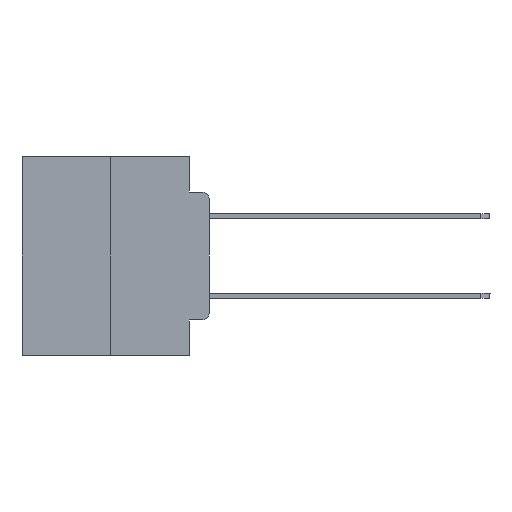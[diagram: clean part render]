
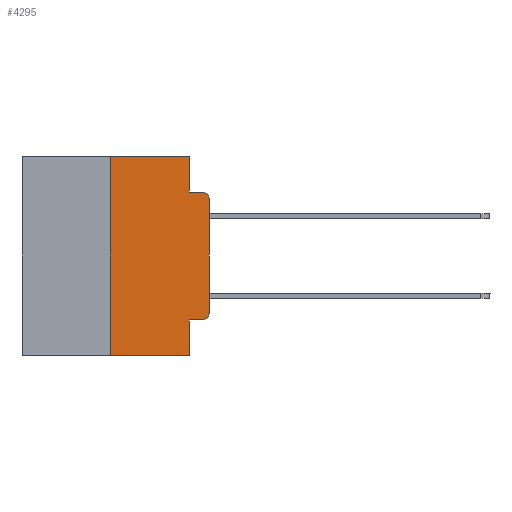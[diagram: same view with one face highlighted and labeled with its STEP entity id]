
A CAD part, left-side view. The second image highlights one B-rep face of the part: STEP entity #4295.
In plain terms, the highlighted planar face has unit normal (-1, 0, 0).
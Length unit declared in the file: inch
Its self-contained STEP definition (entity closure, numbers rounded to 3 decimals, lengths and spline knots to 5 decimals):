
#79 = AXIS2_PLACEMENT_3D ( 'NONE', #15907, #11477, #24116 ) ;
#836 = EDGE_CURVE ( 'NONE', #24686, #2357, #16150, .T. ) ;
#2034 = DIRECTION ( 'NONE',  ( 0., -1., 0. ) ) ;
#2182 = CARTESIAN_POINT ( 'NONE',  ( 0., 0.25, 0. ) ) ;
#2357 = VERTEX_POINT ( 'NONE', #9344 ) ;
#2417 = VECTOR ( 'NONE', #21126, 39.37008 ) ;
#2919 = VECTOR ( 'NONE', #4242, 39.37008 ) ;
#3488 = CIRCLE ( 'NONE', #19843, 0.02 ) ;
#3602 = ORIENTED_EDGE ( 'NONE', *, *, #19411, .F. ) ;
#3713 = DIRECTION ( 'NONE',  ( 0., 0., 1. ) ) ;
#3742 = DIRECTION ( 'NONE',  ( 0., -1., 0. ) ) ;
#3765 = DIRECTION ( 'NONE',  ( 1., 0., 0. ) ) ;
#4242 = DIRECTION ( 'NONE',  ( 0., 0., -1. ) ) ;
#4295 = ADVANCED_FACE ( 'NONE', ( #25111 ), #20653, .F. ) ;
#4565 = VERTEX_POINT ( 'NONE', #24387 ) ;
#4983 = CARTESIAN_POINT ( 'NONE',  ( 0., 0.473, -0.5 ) ) ;
#5387 = CARTESIAN_POINT ( 'NONE',  ( 0., 0., 0. ) ) ;
#5535 = VERTEX_POINT ( 'NONE', #21459 ) ;
#5668 = ORIENTED_EDGE ( 'NONE', *, *, #836, .T. ) ;
#6064 = ORIENTED_EDGE ( 'NONE', *, *, #25754, .T. ) ;
#6255 = ORIENTED_EDGE ( 'NONE', *, *, #13074, .F. ) ;
#6963 = EDGE_CURVE ( 'NONE', #5535, #24871, #11880, .T. ) ;
#7168 = EDGE_CURVE ( 'NONE', #12457, #4565, #27125, .T. ) ;
#7212 = VERTEX_POINT ( 'NONE', #16848 ) ;
#7243 = VECTOR ( 'NONE', #3713, 39.37008 ) ;
#7397 = CARTESIAN_POINT ( 'NONE',  ( 0., 0., -0.1085 ) ) ;
#8178 = VECTOR ( 'NONE', #10061, 39.37008 ) ;
#8630 = LINE ( 'NONE', #19157, #16765 ) ;
#8687 = ORIENTED_EDGE ( 'NONE', *, *, #22724, .T. ) ;
#9344 = CARTESIAN_POINT ( 'NONE',  ( 0., 0.051, -0.5 ) ) ;
#9459 = CARTESIAN_POINT ( 'NONE',  ( 0., 0.051, -0.4115 ) ) ;
#9720 = EDGE_CURVE ( 'NONE', #24686, #15168, #8630, .T. ) ;
#9820 = EDGE_CURVE ( 'NONE', #12457, #2357, #15139, .T. ) ;
#10061 = DIRECTION ( 'NONE',  ( 0., -1., 0. ) ) ;
#10525 = EDGE_CURVE ( 'NONE', #14045, #7212, #22675, .T. ) ;
#11477 = DIRECTION ( 'NONE',  ( -1., 0., 0. ) ) ;
#11880 = LINE ( 'NONE', #5387, #7243 ) ;
#12050 = LINE ( 'NONE', #18420, #20380 ) ;
#12457 = VERTEX_POINT ( 'NONE', #9459 ) ;
#12763 = ORIENTED_EDGE ( 'NONE', *, *, #7168, .T. ) ;
#13074 = EDGE_CURVE ( 'NONE', #15168, #25402, #12050, .T. ) ;
#14045 = VERTEX_POINT ( 'NONE', #24645 ) ;
#14866 = CARTESIAN_POINT ( 'NONE',  ( 0., 0.051, 0. ) ) ;
#15139 = LINE ( 'NONE', #14866, #22537 ) ;
#15168 = VERTEX_POINT ( 'NONE', #2182 ) ;
#15572 = ORIENTED_EDGE ( 'NONE', *, *, #9820, .F. ) ;
#15907 = CARTESIAN_POINT ( 'NONE',  ( 0., 0.02, -0.3915 ) ) ;
#15971 = ORIENTED_EDGE ( 'NONE', *, *, #6963, .T. ) ;
#16150 = LINE ( 'NONE', #4983, #8178 ) ;
#16385 = AXIS2_PLACEMENT_3D ( 'NONE', #25237, #3765, #27173 ) ;
#16717 = CARTESIAN_POINT ( 'NONE',  ( 0., 0.051, -0.4115 ) ) ;
#16765 = VECTOR ( 'NONE', #23182, 39.37008 ) ;
#16848 = CARTESIAN_POINT ( 'NONE',  ( 0., 0.02, -0.0885 ) ) ;
#17257 = LINE ( 'NONE', #23227, #2919 ) ;
#18420 = CARTESIAN_POINT ( 'NONE',  ( 0., 0.473, 0. ) ) ;
#19157 = CARTESIAN_POINT ( 'NONE',  ( 0., 0.25, 0. ) ) ;
#19411 = EDGE_CURVE ( 'NONE', #25402, #14045, #17257, .T. ) ;
#19843 = AXIS2_PLACEMENT_3D ( 'NONE', #20330, #26729, #26458 ) ;
#20330 = CARTESIAN_POINT ( 'NONE',  ( 0., 0.02, -0.1085 ) ) ;
#20380 = VECTOR ( 'NONE', #3742, 39.37008 ) ;
#20512 = VECTOR ( 'NONE', #2034, 39.37008 ) ;
#20653 = PLANE ( 'NONE',  #16385 ) ;
#20917 = CARTESIAN_POINT ( 'NONE',  ( 0., 0.051, 0. ) ) ;
#21126 = DIRECTION ( 'NONE',  ( 0., -1., 0. ) ) ;
#21459 = CARTESIAN_POINT ( 'NONE',  ( 0., 0., -0.3915 ) ) ;
#21768 = CIRCLE ( 'NONE', #79, 0.02 ) ;
#22537 = VECTOR ( 'NONE', #23318, 39.37008 ) ;
#22675 = LINE ( 'NONE', #27106, #2417 ) ;
#22724 = EDGE_CURVE ( 'NONE', #24871, #7212, #3488, .T. ) ;
#22937 = ORIENTED_EDGE ( 'NONE', *, *, #9720, .F. ) ;
#23182 = DIRECTION ( 'NONE',  ( 0., 0., 1. ) ) ;
#23227 = CARTESIAN_POINT ( 'NONE',  ( 0., 0.051, 0. ) ) ;
#23318 = DIRECTION ( 'NONE',  ( 0., 0., -1. ) ) ;
#23626 = CARTESIAN_POINT ( 'NONE',  ( 0., 0.25, -0.5 ) ) ;
#24116 = DIRECTION ( 'NONE',  ( 0., 0., -1. ) ) ;
#24338 = ORIENTED_EDGE ( 'NONE', *, *, #10525, .F. ) ;
#24387 = CARTESIAN_POINT ( 'NONE',  ( 0., 0.02, -0.4115 ) ) ;
#24645 = CARTESIAN_POINT ( 'NONE',  ( 0., 0.051, -0.0885 ) ) ;
#24686 = VERTEX_POINT ( 'NONE', #23626 ) ;
#24822 = EDGE_LOOP ( 'NONE', ( #15971, #8687, #24338, #3602, #6255, #22937, #5668, #15572, #12763, #6064 ) ) ;
#24871 = VERTEX_POINT ( 'NONE', #7397 ) ;
#25111 = FACE_OUTER_BOUND ( 'NONE', #24822, .T. ) ;
#25237 = CARTESIAN_POINT ( 'NONE',  ( 0., 0.473, 0. ) ) ;
#25402 = VERTEX_POINT ( 'NONE', #20917 ) ;
#25754 = EDGE_CURVE ( 'NONE', #4565, #5535, #21768, .T. ) ;
#26458 = DIRECTION ( 'NONE',  ( 0., 0., -1. ) ) ;
#26729 = DIRECTION ( 'NONE',  ( -1., 0., 0. ) ) ;
#27106 = CARTESIAN_POINT ( 'NONE',  ( 0., 0.051, -0.0885 ) ) ;
#27125 = LINE ( 'NONE', #16717, #20512 ) ;
#27173 = DIRECTION ( 'NONE',  ( 0., 0., -1. ) ) ;
